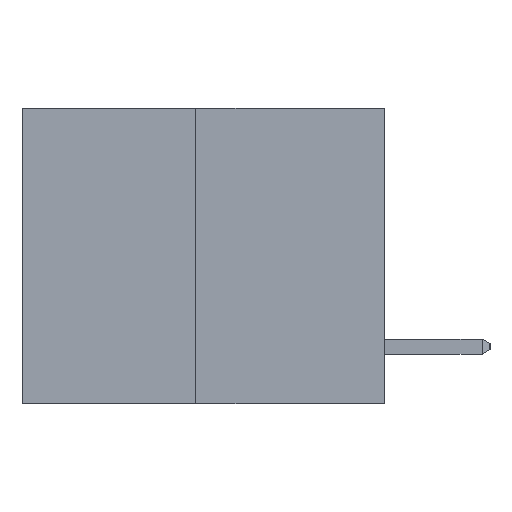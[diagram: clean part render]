
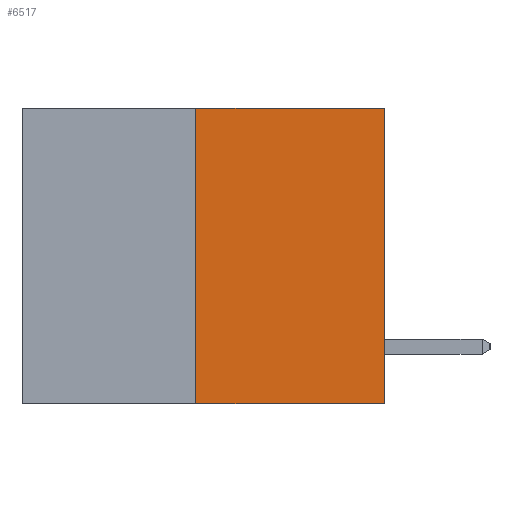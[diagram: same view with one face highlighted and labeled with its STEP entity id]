
A CAD part, left-side view. The second image highlights one B-rep face of the part: STEP entity #6517.
In plain terms, the highlighted planar face has unit normal (-1, 0, 0).
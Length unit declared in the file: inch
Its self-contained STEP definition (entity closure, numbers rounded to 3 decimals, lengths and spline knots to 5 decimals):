
#875 = CARTESIAN_POINT ( 'NONE',  ( 0., 0.312, -0.49 ) ) ;
#913 = VERTEX_POINT ( 'NONE', #15755 ) ;
#1401 = CARTESIAN_POINT ( 'NONE',  ( 0., 0.6, 0. ) ) ;
#1533 = LINE ( 'NONE', #19511, #9720 ) ;
#2689 = EDGE_CURVE ( 'NONE', #4915, #17652, #18681, .T. ) ;
#3221 = ORIENTED_EDGE ( 'NONE', *, *, #6859, .T. ) ;
#3991 = DIRECTION ( 'NONE',  ( 0., 0., 1. ) ) ;
#4666 = DIRECTION ( 'NONE',  ( 0., -1., 0. ) ) ;
#4915 = VERTEX_POINT ( 'NONE', #875 ) ;
#5272 = CARTESIAN_POINT ( 'NONE',  ( 0., 0., 0. ) ) ;
#5808 = DIRECTION ( 'NONE',  ( 0., -1., 0. ) ) ;
#5901 = VECTOR ( 'NONE', #11547, 39.37008 ) ;
#6311 = VECTOR ( 'NONE', #4666, 39.37008 ) ;
#6517 = ADVANCED_FACE ( 'NONE', ( #11895 ), #9865, .F. ) ;
#6859 = EDGE_CURVE ( 'NONE', #17652, #20236, #1533, .T. ) ;
#7331 = ORIENTED_EDGE ( 'NONE', *, *, #2689, .T. ) ;
#9720 = VECTOR ( 'NONE', #3991, 39.37008 ) ;
#9865 = PLANE ( 'NONE',  #13619 ) ;
#10559 = EDGE_LOOP ( 'NONE', ( #12168, #7331, #3221, #20384 ) ) ;
#11547 = DIRECTION ( 'NONE',  ( 0., 0., 1. ) ) ;
#11728 = LINE ( 'NONE', #15551, #6311 ) ;
#11895 = FACE_OUTER_BOUND ( 'NONE', #10559, .T. ) ;
#12168 = ORIENTED_EDGE ( 'NONE', *, *, #21917, .F. ) ;
#13548 = LINE ( 'NONE', #20389, #5901 ) ;
#13592 = CARTESIAN_POINT ( 'NONE',  ( 0., 0., -0.49 ) ) ;
#13619 = AXIS2_PLACEMENT_3D ( 'NONE', #1401, #15437, #16884 ) ;
#14061 = VECTOR ( 'NONE', #5808, 39.37008 ) ;
#14273 = CARTESIAN_POINT ( 'NONE',  ( 0., 0.6, -0.49 ) ) ;
#14650 = EDGE_CURVE ( 'NONE', #913, #20236, #11728, .T. ) ;
#15437 = DIRECTION ( 'NONE',  ( 1., 0., 0. ) ) ;
#15551 = CARTESIAN_POINT ( 'NONE',  ( 0., 0.6, 0. ) ) ;
#15755 = CARTESIAN_POINT ( 'NONE',  ( 0., 0.312, 0. ) ) ;
#16884 = DIRECTION ( 'NONE',  ( 0., 0., -1. ) ) ;
#17652 = VERTEX_POINT ( 'NONE', #13592 ) ;
#18681 = LINE ( 'NONE', #14273, #14061 ) ;
#19511 = CARTESIAN_POINT ( 'NONE',  ( 0., 0., 0. ) ) ;
#20236 = VERTEX_POINT ( 'NONE', #5272 ) ;
#20384 = ORIENTED_EDGE ( 'NONE', *, *, #14650, .F. ) ;
#20389 = CARTESIAN_POINT ( 'NONE',  ( 0., 0.312, -0.49 ) ) ;
#21917 = EDGE_CURVE ( 'NONE', #4915, #913, #13548, .T. ) ;
